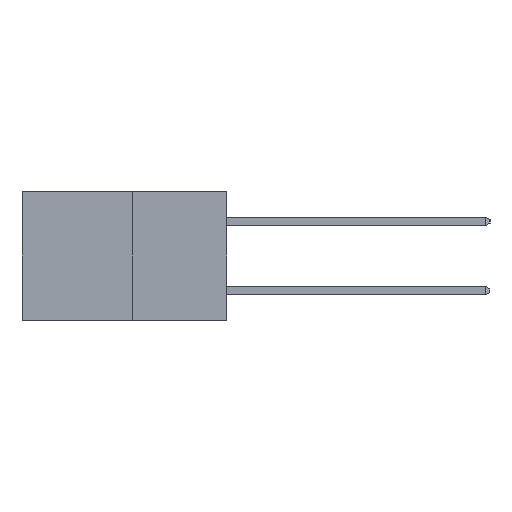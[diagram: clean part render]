
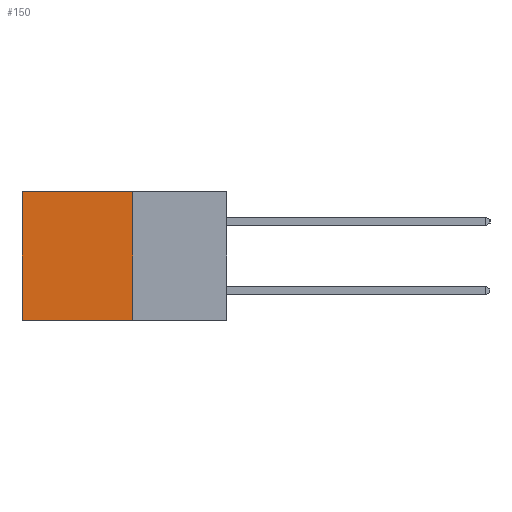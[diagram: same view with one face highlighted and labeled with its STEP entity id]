
A CAD part, left-side view. The second image highlights one B-rep face of the part: STEP entity #150.
In plain terms, the highlighted planar face has unit normal (-1, 0, 0).
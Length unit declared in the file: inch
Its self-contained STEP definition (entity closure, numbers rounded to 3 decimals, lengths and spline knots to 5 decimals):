
#150 = ADVANCED_FACE ( 'NONE', ( #10126 ), #4275, .F. ) ;
#168 = VECTOR ( 'NONE', #2325, 39.37008 ) ;
#724 = VERTEX_POINT ( 'NONE', #8071 ) ;
#1262 = CARTESIAN_POINT ( 'NONE',  ( 0.277, 0.27, -0.37 ) ) ;
#1393 = CARTESIAN_POINT ( 'NONE',  ( 0.277, 0.59, 0. ) ) ;
#1406 = DIRECTION ( 'NONE',  ( 0., 0., -1. ) ) ;
#2325 = DIRECTION ( 'NONE',  ( 0., 1., 0. ) ) ;
#2640 = EDGE_CURVE ( 'NONE', #724, #2726, #6268, .T. ) ;
#2726 = VERTEX_POINT ( 'NONE', #1393 ) ;
#3611 = VECTOR ( 'NONE', #9463, 39.37008 ) ;
#3699 = DIRECTION ( 'NONE',  ( 0., 0., -1. ) ) ;
#4275 = PLANE ( 'NONE',  #4905 ) ;
#4557 = DIRECTION ( 'NONE',  ( 1., 0., 0. ) ) ;
#4813 = ORIENTED_EDGE ( 'NONE', *, *, #13967, .F. ) ;
#4905 = AXIS2_PLACEMENT_3D ( 'NONE', #5725, #4557, #3699 ) ;
#5725 = CARTESIAN_POINT ( 'NONE',  ( 0.277, 0.27, -0.37 ) ) ;
#6268 = LINE ( 'NONE', #9603, #168 ) ;
#6621 = LINE ( 'NONE', #10609, #3611 ) ;
#6778 = DIRECTION ( 'NONE',  ( 0., 0., -1. ) ) ;
#7194 = LINE ( 'NONE', #9411, #13204 ) ;
#7319 = VECTOR ( 'NONE', #6778, 39.37008 ) ;
#7843 = ORIENTED_EDGE ( 'NONE', *, *, #2640, .T. ) ;
#8071 = CARTESIAN_POINT ( 'NONE',  ( 0.277, 0.27, 0. ) ) ;
#8437 = EDGE_CURVE ( 'NONE', #11661, #9771, #6621, .T. ) ;
#8854 = EDGE_CURVE ( 'NONE', #2726, #9771, #10385, .T. ) ;
#9411 = CARTESIAN_POINT ( 'NONE',  ( 0.277, 0.27, -0.37 ) ) ;
#9463 = DIRECTION ( 'NONE',  ( 0., 1., 0. ) ) ;
#9603 = CARTESIAN_POINT ( 'NONE',  ( 0.277, 0.27, 0. ) ) ;
#9771 = VERTEX_POINT ( 'NONE', #13819 ) ;
#10126 = FACE_OUTER_BOUND ( 'NONE', #10692, .T. ) ;
#10385 = LINE ( 'NONE', #11337, #7319 ) ;
#10609 = CARTESIAN_POINT ( 'NONE',  ( 0.277, 0.27, -0.37 ) ) ;
#10692 = EDGE_LOOP ( 'NONE', ( #12054, #13349, #4813, #7843 ) ) ;
#11337 = CARTESIAN_POINT ( 'NONE',  ( 0.277, 0.59, -0.37 ) ) ;
#11661 = VERTEX_POINT ( 'NONE', #1262 ) ;
#12054 = ORIENTED_EDGE ( 'NONE', *, *, #8854, .T. ) ;
#13204 = VECTOR ( 'NONE', #1406, 39.37008 ) ;
#13349 = ORIENTED_EDGE ( 'NONE', *, *, #8437, .F. ) ;
#13819 = CARTESIAN_POINT ( 'NONE',  ( 0.277, 0.59, -0.37 ) ) ;
#13967 = EDGE_CURVE ( 'NONE', #724, #11661, #7194, .T. ) ;
